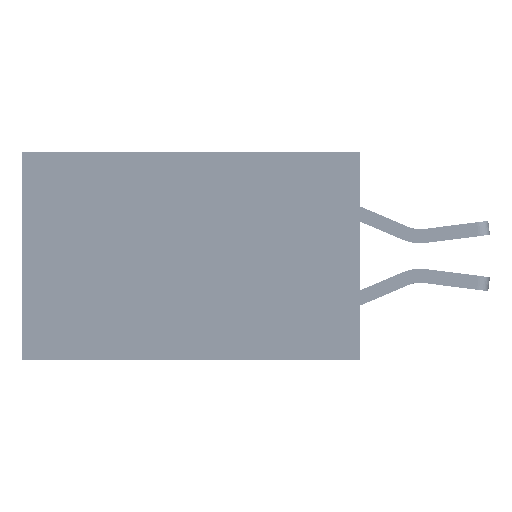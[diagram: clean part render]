
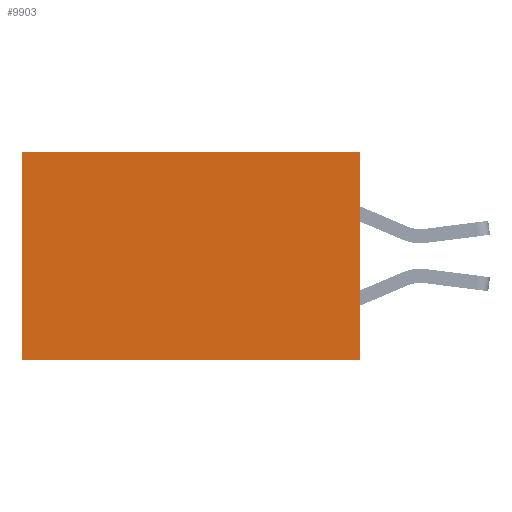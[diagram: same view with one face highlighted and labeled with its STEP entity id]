
A CAD part, left-side view. The second image highlights one B-rep face of the part: STEP entity #9903.
In plain terms, the highlighted planar face has unit normal (-1, 0, 0).
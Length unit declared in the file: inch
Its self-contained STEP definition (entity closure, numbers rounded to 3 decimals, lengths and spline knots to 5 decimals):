
#909 = DIRECTION ( 'NONE',  ( 1., 0., 0. ) ) ;
#2084 = ORIENTED_EDGE ( 'NONE', *, *, #6820, .T. ) ;
#3357 = DIRECTION ( 'NONE',  ( 0., 1., 0. ) ) ;
#4238 = CARTESIAN_POINT ( 'NONE',  ( 0.2875, 0., 0. ) ) ;
#6542 = LINE ( 'NONE', #33733, #37035 ) ;
#6820 = EDGE_CURVE ( 'NONE', #28539, #18798, #13113, .T. ) ;
#7922 = VECTOR ( 'NONE', #33204, 39.37008 ) ;
#9903 = ADVANCED_FACE ( 'NONE', ( #18456 ), #16473, .F. ) ;
#13113 = LINE ( 'NONE', #37169, #27885 ) ;
#14170 = EDGE_CURVE ( 'NONE', #18798, #36611, #6542, .T. ) ;
#14530 = DIRECTION ( 'NONE',  ( 0., 0., -1. ) ) ;
#15083 = ORIENTED_EDGE ( 'NONE', *, *, #14170, .T. ) ;
#15697 = DIRECTION ( 'NONE',  ( 0., 0., -1. ) ) ;
#16473 = PLANE ( 'NONE',  #31939 ) ;
#16982 = CARTESIAN_POINT ( 'NONE',  ( 0.2875, 0., -0.37 ) ) ;
#18456 = FACE_OUTER_BOUND ( 'NONE', #28226, .T. ) ;
#18798 = VERTEX_POINT ( 'NONE', #32949 ) ;
#19522 = DIRECTION ( 'NONE',  ( 0., 1., 0. ) ) ;
#22835 = LINE ( 'NONE', #37195, #37583 ) ;
#24580 = EDGE_CURVE ( 'NONE', #34376, #36611, #22835, .T. ) ;
#24981 = LINE ( 'NONE', #36312, #7922 ) ;
#27885 = VECTOR ( 'NONE', #19522, 39.37008 ) ;
#28226 = EDGE_LOOP ( 'NONE', ( #15083, #29198, #33283, #2084 ) ) ;
#28539 = VERTEX_POINT ( 'NONE', #34343 ) ;
#29198 = ORIENTED_EDGE ( 'NONE', *, *, #24580, .F. ) ;
#30274 = CARTESIAN_POINT ( 'NONE',  ( 0.2875, 0.6, -0.37 ) ) ;
#31939 = AXIS2_PLACEMENT_3D ( 'NONE', #4238, #909, #14530 ) ;
#32949 = CARTESIAN_POINT ( 'NONE',  ( 0.2875, 0.6, 0. ) ) ;
#33204 = DIRECTION ( 'NONE',  ( 0., 0., -1. ) ) ;
#33283 = ORIENTED_EDGE ( 'NONE', *, *, #36021, .F. ) ;
#33733 = CARTESIAN_POINT ( 'NONE',  ( 0.2875, 0.6, 0. ) ) ;
#34343 = CARTESIAN_POINT ( 'NONE',  ( 0.2875, 0., 0. ) ) ;
#34376 = VERTEX_POINT ( 'NONE', #16982 ) ;
#36021 = EDGE_CURVE ( 'NONE', #28539, #34376, #24981, .T. ) ;
#36312 = CARTESIAN_POINT ( 'NONE',  ( 0.2875, 0., 0. ) ) ;
#36611 = VERTEX_POINT ( 'NONE', #30274 ) ;
#37035 = VECTOR ( 'NONE', #15697, 39.37008 ) ;
#37169 = CARTESIAN_POINT ( 'NONE',  ( 0.2875, 0., 0. ) ) ;
#37195 = CARTESIAN_POINT ( 'NONE',  ( 0.2875, 0., -0.37 ) ) ;
#37583 = VECTOR ( 'NONE', #3357, 39.37008 ) ;
